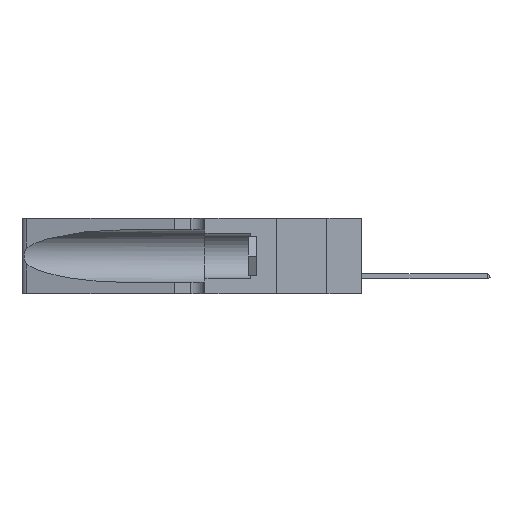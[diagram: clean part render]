
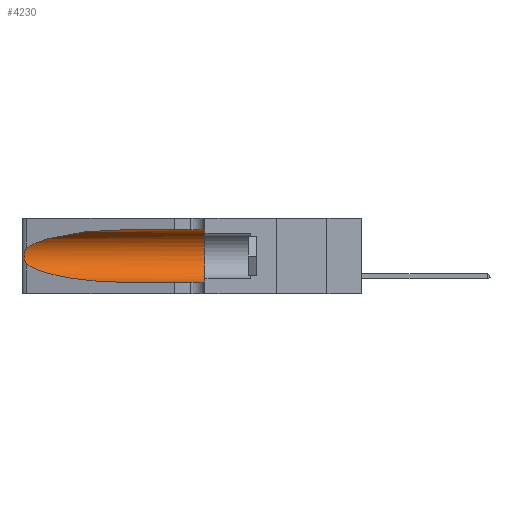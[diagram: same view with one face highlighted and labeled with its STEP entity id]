
A CAD part, left-side view. The second image highlights one B-rep face of the part: STEP entity #4230.
In plain terms, the highlighted cylindrical face has radius 3.308 mm (diameter 6.617 mm), a partial arc.
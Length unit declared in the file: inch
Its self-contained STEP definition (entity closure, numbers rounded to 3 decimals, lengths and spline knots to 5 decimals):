
#81 = DIRECTION ( 'NONE',  ( 0., 1., 0. ) ) ;
#158 =( BOUNDED_CURVE ( )  B_SPLINE_CURVE ( 3, ( #2446, #14578, #16206, #4396 ),
 .UNSPECIFIED., .F., .F. ) 
 B_SPLINE_CURVE_WITH_KNOTS ( ( 4, 4 ),
 ( 3.44316, 4.71239 ),
 .UNSPECIFIED. ) 
 CURVE ( )  GEOMETRIC_REPRESENTATION_ITEM ( )  RATIONAL_B_SPLINE_CURVE ( ( 1., 0.87, 0.87, 1. ) ) 
 REPRESENTATION_ITEM ( '' )  );
#555 = CARTESIAN_POINT ( 'NONE',  ( 0.25555, 1.22993, 0.14849 ) ) ;
#695 = CARTESIAN_POINT ( 'NONE',  ( 0.1305, 0.72297, 0.31525 ) ) ;
#1448 = VERTEX_POINT ( 'NONE', #1449 ) ;
#1449 = CARTESIAN_POINT ( 'NONE',  ( 0.1305, 0.35, 0.05475 ) ) ;
#2061 = CARTESIAN_POINT ( 'NONE',  ( 0.26075, 1.23896, 0.178 ) ) ;
#2378 = CARTESIAN_POINT ( 'NONE',  ( 0.25487, 1.22718, 0.14631 ) ) ;
#2421 = CYLINDRICAL_SURFACE ( 'NONE', #19973, 0.13025 ) ;
#2446 = CARTESIAN_POINT ( 'NONE',  ( 0.25487, 1.22718, 0.14631 ) ) ;
#3265 = EDGE_LOOP ( 'NONE', ( #20604, #13844, #7918, #13916, #5026, #19221 ) ) ;
#3680 = EDGE_CURVE ( 'NONE', #4965, #1448, #15510, .T. ) ;
#4113 = CARTESIAN_POINT ( 'NONE',  ( 0.25639, 1.23184, 0.21858 ) ) ;
#4230 = ADVANCED_FACE ( 'NONE', ( #8548 ), #2421, .F. ) ;
#4307 = CARTESIAN_POINT ( 'NONE',  ( 0.25487, 1.22718, 0.22369 ) ) ;
#4396 = CARTESIAN_POINT ( 'NONE',  ( 0.1305, 0.72297, 0.05475 ) ) ;
#4965 = VERTEX_POINT ( 'NONE', #17124 ) ;
#5026 = ORIENTED_EDGE ( 'NONE', *, *, #10286, .F. ) ;
#5218 = CARTESIAN_POINT ( 'NONE',  ( 0.1305, 0.35, 0.185 ) ) ;
#7236 = CARTESIAN_POINT ( 'NONE',  ( 0.25854, 1.2359, 0.20912 ) ) ;
#7373 = CARTESIAN_POINT ( 'NONE',  ( 0.25787, 1.23484, 0.2124 ) ) ;
#7701 = DIRECTION ( 'NONE',  ( 0., 0., -1. ) ) ;
#7737 = LINE ( 'NONE', #19050, #8018 ) ;
#7918 = ORIENTED_EDGE ( 'NONE', *, *, #8039, .T. ) ;
#8018 = VECTOR ( 'NONE', #8821, 39.37008 ) ;
#8039 = EDGE_CURVE ( 'NONE', #19451, #4965, #158, .T. ) ;
#8252 = B_SPLINE_CURVE_WITH_KNOTS ( 'NONE', 3,
 ( #12334, #12261, #4113, #7373, #7236, #17423, #9102, #2061, #12562, #17726, #21066, #14280, #555, #2378 ),
 .UNSPECIFIED., .F., .F.,
 ( 4, 2, 2, 2, 2, 2, 4 ),
 ( 0., 0.00027, 0.00053, 0.00107, 0.0016, 0.00187, 0.00214 ),
 .UNSPECIFIED. ) ;
#8548 = FACE_OUTER_BOUND ( 'NONE', #3265, .T. ) ;
#8821 = DIRECTION ( 'NONE',  ( 0., -1., 0. ) ) ;
#8991 = CARTESIAN_POINT ( 'NONE',  ( 0.1305, 1.61858, 0.05475 ) ) ;
#9102 = CARTESIAN_POINT ( 'NONE',  ( 0.26075, 1.23896, 0.19203 ) ) ;
#9383 = CARTESIAN_POINT ( 'NONE',  ( 0.25487, 1.22718, 0.22369 ) ) ;
#9559 = CARTESIAN_POINT ( 'NONE',  ( 0.1305, 1.61858, 0.185 ) ) ;
#10286 = EDGE_CURVE ( 'NONE', #20705, #1448, #15181, .T. ) ;
#10439 = EDGE_CURVE ( 'NONE', #19991, #16559, #16158, .T. ) ;
#10632 = EDGE_CURVE ( 'NONE', #19991, #20705, #7737, .T. ) ;
#11260 = DIRECTION ( 'NONE',  ( 0., -1., 0. ) ) ;
#12261 = CARTESIAN_POINT ( 'NONE',  ( 0.25555, 1.22994, 0.2215 ) ) ;
#12334 = CARTESIAN_POINT ( 'NONE',  ( 0.25487, 1.22718, 0.22369 ) ) ;
#12562 = CARTESIAN_POINT ( 'NONE',  ( 0.26017, 1.23833, 0.17102 ) ) ;
#13844 = ORIENTED_EDGE ( 'NONE', *, *, #16356, .T. ) ;
#13916 = ORIENTED_EDGE ( 'NONE', *, *, #3680, .T. ) ;
#14251 = DIRECTION ( 'NONE',  ( 0., -1., 0. ) ) ;
#14280 = CARTESIAN_POINT ( 'NONE',  ( 0.25639, 1.23186, 0.15144 ) ) ;
#14578 = CARTESIAN_POINT ( 'NONE',  ( 0.2373, 1.15595, 0.08982 ) ) ;
#15142 = AXIS2_PLACEMENT_3D ( 'NONE', #5218, #81, #18862 ) ;
#15181 = CIRCLE ( 'NONE', #15142, 0.13025 ) ;
#15510 = LINE ( 'NONE', #8991, #21722 ) ;
#16158 =( BOUNDED_CURVE ( )  B_SPLINE_CURVE ( 3, ( #695, #19678, #16267, #4307 ),
 .UNSPECIFIED., .F., .F. ) 
 B_SPLINE_CURVE_WITH_KNOTS ( ( 4, 4 ),
 ( 1.5708, 2.84003 ),
 .UNSPECIFIED. ) 
 CURVE ( )  GEOMETRIC_REPRESENTATION_ITEM ( )  RATIONAL_B_SPLINE_CURVE ( ( 1., 0.87, 0.87, 1. ) ) 
 REPRESENTATION_ITEM ( '' )  );
#16206 = CARTESIAN_POINT ( 'NONE',  ( 0.18966, 0.96281, 0.05475 ) ) ;
#16267 = CARTESIAN_POINT ( 'NONE',  ( 0.2373, 1.15595, 0.28018 ) ) ;
#16356 = EDGE_CURVE ( 'NONE', #16559, #19451, #8252, .T. ) ;
#16559 = VERTEX_POINT ( 'NONE', #9383 ) ;
#16902 = CARTESIAN_POINT ( 'NONE',  ( 0.25487, 1.22718, 0.14631 ) ) ;
#16997 = CARTESIAN_POINT ( 'NONE',  ( 0.1305, 0.72297, 0.31525 ) ) ;
#17124 = CARTESIAN_POINT ( 'NONE',  ( 0.1305, 0.72297, 0.05475 ) ) ;
#17423 = CARTESIAN_POINT ( 'NONE',  ( 0.26018, 1.23835, 0.19895 ) ) ;
#17726 = CARTESIAN_POINT ( 'NONE',  ( 0.25856, 1.23593, 0.16098 ) ) ;
#18862 = DIRECTION ( 'NONE',  ( 0., 0., 1. ) ) ;
#19050 = CARTESIAN_POINT ( 'NONE',  ( 0.1305, 1.61858, 0.31525 ) ) ;
#19221 = ORIENTED_EDGE ( 'NONE', *, *, #10632, .F. ) ;
#19451 = VERTEX_POINT ( 'NONE', #16902 ) ;
#19678 = CARTESIAN_POINT ( 'NONE',  ( 0.18966, 0.96281, 0.31525 ) ) ;
#19973 = AXIS2_PLACEMENT_3D ( 'NONE', #9559, #11260, #7701 ) ;
#19991 = VERTEX_POINT ( 'NONE', #16997 ) ;
#20604 = ORIENTED_EDGE ( 'NONE', *, *, #10439, .T. ) ;
#20705 = VERTEX_POINT ( 'NONE', #22175 ) ;
#21066 = CARTESIAN_POINT ( 'NONE',  ( 0.25789, 1.23486, 0.15765 ) ) ;
#21722 = VECTOR ( 'NONE', #14251, 39.37008 ) ;
#22175 = CARTESIAN_POINT ( 'NONE',  ( 0.1305, 0.35, 0.31525 ) ) ;
